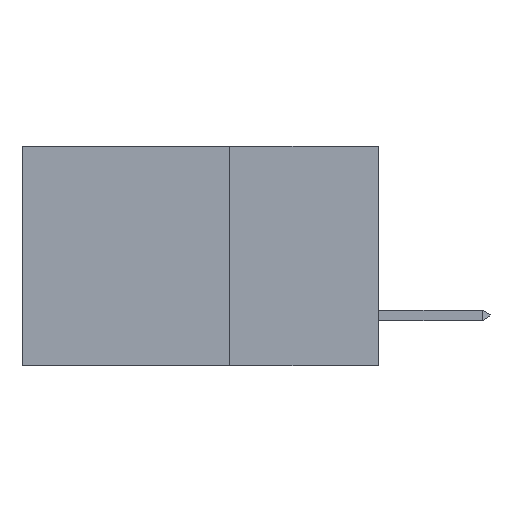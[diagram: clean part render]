
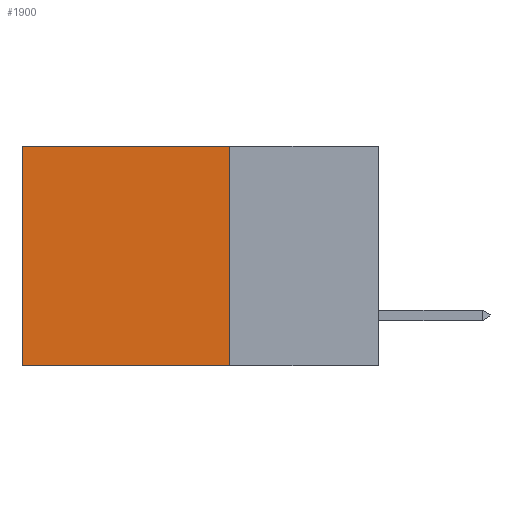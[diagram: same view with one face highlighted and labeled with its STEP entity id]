
A CAD part, left-side view. The second image highlights one B-rep face of the part: STEP entity #1900.
In plain terms, the highlighted planar face has unit normal (-1, 0, 0).
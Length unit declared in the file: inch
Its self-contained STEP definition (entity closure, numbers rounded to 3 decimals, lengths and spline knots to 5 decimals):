
#49 = DIRECTION ( 'NONE',  ( 1., 0., 0. ) ) ;
#628 = DIRECTION ( 'NONE',  ( 0., 1., 0. ) ) ;
#1814 = VERTEX_POINT ( 'NONE', #13586 ) ;
#1900 = ADVANCED_FACE ( 'NONE', ( #17465 ), #19146, .F. ) ;
#2173 = CARTESIAN_POINT ( 'NONE',  ( 0.2615, 0.25, 0. ) ) ;
#2329 = LINE ( 'NONE', #13642, #6881 ) ;
#2673 = LINE ( 'NONE', #2173, #17503 ) ;
#2970 = AXIS2_PLACEMENT_3D ( 'NONE', #6263, #49, #12816 ) ;
#3247 = VECTOR ( 'NONE', #18097, 39.37008 ) ;
#3894 = LINE ( 'NONE', #19561, #3247 ) ;
#3905 = VERTEX_POINT ( 'NONE', #6006 ) ;
#3924 = ORIENTED_EDGE ( 'NONE', *, *, #12282, .F. ) ;
#6006 = CARTESIAN_POINT ( 'NONE',  ( 0.2615, 0.25, 0. ) ) ;
#6263 = CARTESIAN_POINT ( 'NONE',  ( 0.2615, 0.25, -0.37 ) ) ;
#6881 = VECTOR ( 'NONE', #10326, 39.37008 ) ;
#7014 = EDGE_CURVE ( 'NONE', #3905, #9649, #14221, .T. ) ;
#9649 = VERTEX_POINT ( 'NONE', #11046 ) ;
#10206 = VECTOR ( 'NONE', #12565, 39.37008 ) ;
#10326 = DIRECTION ( 'NONE',  ( 0., 0., -1. ) ) ;
#10549 = EDGE_LOOP ( 'NONE', ( #13206, #3924, #11142, #16255 ) ) ;
#11046 = CARTESIAN_POINT ( 'NONE',  ( 0.2615, 0.25, -0.37 ) ) ;
#11142 = ORIENTED_EDGE ( 'NONE', *, *, #7014, .F. ) ;
#12217 = EDGE_CURVE ( 'NONE', #14396, #1814, #2329, .T. ) ;
#12282 = EDGE_CURVE ( 'NONE', #9649, #1814, #3894, .T. ) ;
#12565 = DIRECTION ( 'NONE',  ( 0., 0., -1. ) ) ;
#12816 = DIRECTION ( 'NONE',  ( 0., 0., -1. ) ) ;
#13206 = ORIENTED_EDGE ( 'NONE', *, *, #12217, .T. ) ;
#13270 = EDGE_CURVE ( 'NONE', #3905, #14396, #2673, .T. ) ;
#13586 = CARTESIAN_POINT ( 'NONE',  ( 0.2615, 0.6, -0.37 ) ) ;
#13642 = CARTESIAN_POINT ( 'NONE',  ( 0.2615, 0.6, -0.37 ) ) ;
#14017 = CARTESIAN_POINT ( 'NONE',  ( 0.2615, 0.25, -0.37 ) ) ;
#14221 = LINE ( 'NONE', #14017, #10206 ) ;
#14396 = VERTEX_POINT ( 'NONE', #18281 ) ;
#16255 = ORIENTED_EDGE ( 'NONE', *, *, #13270, .T. ) ;
#17465 = FACE_OUTER_BOUND ( 'NONE', #10549, .T. ) ;
#17503 = VECTOR ( 'NONE', #628, 39.37008 ) ;
#18097 = DIRECTION ( 'NONE',  ( 0., 1., 0. ) ) ;
#18281 = CARTESIAN_POINT ( 'NONE',  ( 0.2615, 0.6, 0. ) ) ;
#19146 = PLANE ( 'NONE',  #2970 ) ;
#19561 = CARTESIAN_POINT ( 'NONE',  ( 0.2615, 0.25, -0.37 ) ) ;
